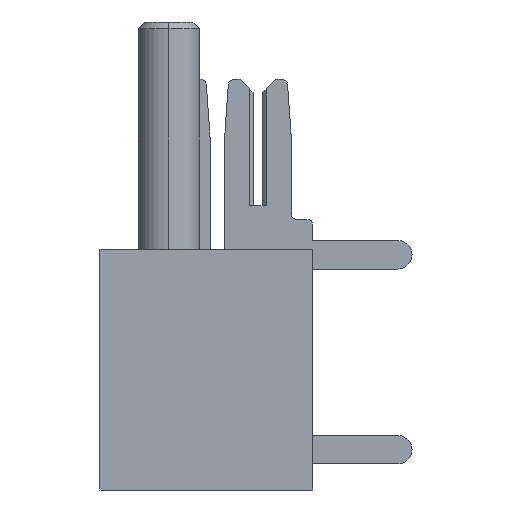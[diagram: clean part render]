
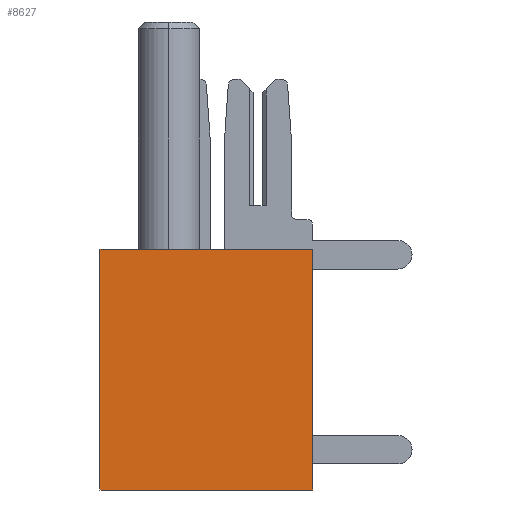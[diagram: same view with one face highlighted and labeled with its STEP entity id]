
A CAD part, left-side view. The second image highlights one B-rep face of the part: STEP entity #8627.
In plain terms, the highlighted planar face has unit normal (-1, 0, 0).
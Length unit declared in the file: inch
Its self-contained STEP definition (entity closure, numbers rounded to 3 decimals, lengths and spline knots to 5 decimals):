
#89 = EDGE_LOOP ( 'NONE', ( #6863, #10973, #8162, #6296 ) ) ;
#288 = CARTESIAN_POINT ( 'NONE',  ( 0., 0., 0. ) ) ;
#1061 = AXIS2_PLACEMENT_3D ( 'NONE', #11682, #8771, #11636 ) ;
#1570 = VERTEX_POINT ( 'NONE', #6381 ) ;
#1684 = DIRECTION ( 'NONE',  ( 0., -1., 0. ) ) ;
#1728 = CARTESIAN_POINT ( 'NONE',  ( 0., 0., -0.37 ) ) ;
#2238 = LINE ( 'NONE', #288, #6481 ) ;
#2265 = CARTESIAN_POINT ( 'NONE',  ( 0., 0.327, 0. ) ) ;
#2461 = DIRECTION ( 'NONE',  ( 0., 0., 1. ) ) ;
#3124 = PLANE ( 'NONE',  #1061 ) ;
#3415 = CARTESIAN_POINT ( 'NONE',  ( 0., 0.327, -0.37 ) ) ;
#4103 = VECTOR ( 'NONE', #1684, 39.37008 ) ;
#5323 = VERTEX_POINT ( 'NONE', #9597 ) ;
#6296 = ORIENTED_EDGE ( 'NONE', *, *, #11589, .T. ) ;
#6381 = CARTESIAN_POINT ( 'NONE',  ( 0., 0.327, -0.37 ) ) ;
#6481 = VECTOR ( 'NONE', #11812, 39.37008 ) ;
#6784 = VECTOR ( 'NONE', #12005, 39.37008 ) ;
#6863 = ORIENTED_EDGE ( 'NONE', *, *, #7500, .F. ) ;
#7500 = EDGE_CURVE ( 'NONE', #7594, #5323, #2238, .T. ) ;
#7527 = FACE_OUTER_BOUND ( 'NONE', #89, .T. ) ;
#7594 = VERTEX_POINT ( 'NONE', #2265 ) ;
#7702 = EDGE_CURVE ( 'NONE', #1570, #7594, #9311, .T. ) ;
#8162 = ORIENTED_EDGE ( 'NONE', *, *, #10897, .T. ) ;
#8166 = VECTOR ( 'NONE', #2461, 39.37008 ) ;
#8193 = LINE ( 'NONE', #1728, #4103 ) ;
#8451 = LINE ( 'NONE', #11081, #8166 ) ;
#8627 = ADVANCED_FACE ( 'NONE', ( #7527 ), #3124, .T. ) ;
#8771 = DIRECTION ( 'NONE',  ( -1., 0., 0. ) ) ;
#9311 = LINE ( 'NONE', #3415, #6784 ) ;
#9597 = CARTESIAN_POINT ( 'NONE',  ( 0., 0., 0. ) ) ;
#10897 = EDGE_CURVE ( 'NONE', #1570, #11920, #8193, .T. ) ;
#10973 = ORIENTED_EDGE ( 'NONE', *, *, #7702, .F. ) ;
#11081 = CARTESIAN_POINT ( 'NONE',  ( 0., 0., -0.37 ) ) ;
#11356 = CARTESIAN_POINT ( 'NONE',  ( 0., 0., -0.37 ) ) ;
#11589 = EDGE_CURVE ( 'NONE', #11920, #5323, #8451, .T. ) ;
#11636 = DIRECTION ( 'NONE',  ( 0., 0., 1. ) ) ;
#11682 = CARTESIAN_POINT ( 'NONE',  ( 0., 0., -0.37 ) ) ;
#11812 = DIRECTION ( 'NONE',  ( 0., -1., 0. ) ) ;
#11920 = VERTEX_POINT ( 'NONE', #11356 ) ;
#12005 = DIRECTION ( 'NONE',  ( 0., 0., 1. ) ) ;
